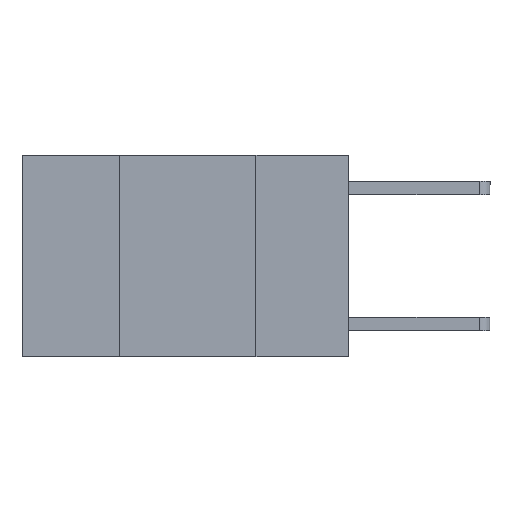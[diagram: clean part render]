
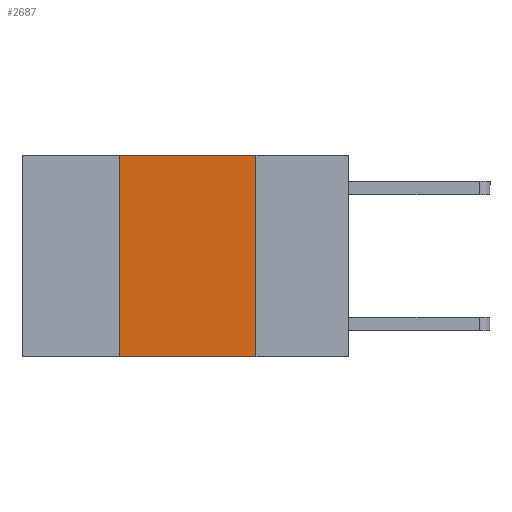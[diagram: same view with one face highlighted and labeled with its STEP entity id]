
A CAD part, left-side view. The second image highlights one B-rep face of the part: STEP entity #2687.
In plain terms, the highlighted planar face has unit normal (-1, 0, 0).
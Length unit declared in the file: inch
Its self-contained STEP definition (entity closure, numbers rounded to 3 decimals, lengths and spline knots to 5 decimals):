
#352 = FACE_OUTER_BOUND ( 'NONE', #5552, .T. ) ;
#398 = ORIENTED_EDGE ( 'NONE', *, *, #6599, .F. ) ;
#625 = VECTOR ( 'NONE', #4652, 39.37008 ) ;
#720 = LINE ( 'NONE', #4434, #6132 ) ;
#852 = LINE ( 'NONE', #4531, #5296 ) ;
#1449 = VERTEX_POINT ( 'NONE', #8248 ) ;
#1647 = CARTESIAN_POINT ( 'NONE',  ( 0., 0.6, 0. ) ) ;
#2238 = VECTOR ( 'NONE', #4436, 39.37008 ) ;
#2485 = LINE ( 'NONE', #7706, #2238 ) ;
#2576 = VERTEX_POINT ( 'NONE', #3418 ) ;
#2687 = ADVANCED_FACE ( 'NONE', ( #352 ), #4977, .F. ) ;
#2700 = CARTESIAN_POINT ( 'NONE',  ( 0., 0.6, -0.37 ) ) ;
#2805 = EDGE_CURVE ( 'NONE', #2576, #2960, #2485, .T. ) ;
#2960 = VERTEX_POINT ( 'NONE', #5774 ) ;
#3195 = CARTESIAN_POINT ( 'NONE',  ( 0., 0.17, -0.37 ) ) ;
#3418 = CARTESIAN_POINT ( 'NONE',  ( 0., 0.42, -0.37 ) ) ;
#3520 = EDGE_CURVE ( 'NONE', #2576, #6836, #7166, .T. ) ;
#3794 = EDGE_CURVE ( 'NONE', #1449, #6836, #720, .T. ) ;
#4040 = AXIS2_PLACEMENT_3D ( 'NONE', #1647, #4310, #6175 ) ;
#4310 = DIRECTION ( 'NONE',  ( 1., 0., 0. ) ) ;
#4434 = CARTESIAN_POINT ( 'NONE',  ( 0., 0.17, 0. ) ) ;
#4436 = DIRECTION ( 'NONE',  ( 0., 0., 1. ) ) ;
#4516 = DIRECTION ( 'NONE',  ( 0., 0., -1. ) ) ;
#4531 = CARTESIAN_POINT ( 'NONE',  ( 0., 0.6, 0. ) ) ;
#4652 = DIRECTION ( 'NONE',  ( 0., -1., 0. ) ) ;
#4977 = PLANE ( 'NONE',  #4040 ) ;
#5296 = VECTOR ( 'NONE', #7090, 39.37008 ) ;
#5552 = EDGE_LOOP ( 'NONE', ( #7351, #398, #6984, #6915 ) ) ;
#5774 = CARTESIAN_POINT ( 'NONE',  ( 0., 0.42, 0. ) ) ;
#6132 = VECTOR ( 'NONE', #4516, 39.37008 ) ;
#6175 = DIRECTION ( 'NONE',  ( 0., 0., -1. ) ) ;
#6599 = EDGE_CURVE ( 'NONE', #2960, #1449, #852, .T. ) ;
#6836 = VERTEX_POINT ( 'NONE', #3195 ) ;
#6915 = ORIENTED_EDGE ( 'NONE', *, *, #3520, .T. ) ;
#6984 = ORIENTED_EDGE ( 'NONE', *, *, #2805, .F. ) ;
#7090 = DIRECTION ( 'NONE',  ( 0., -1., 0. ) ) ;
#7166 = LINE ( 'NONE', #2700, #625 ) ;
#7351 = ORIENTED_EDGE ( 'NONE', *, *, #3794, .F. ) ;
#7706 = CARTESIAN_POINT ( 'NONE',  ( 0., 0.42, 0. ) ) ;
#8248 = CARTESIAN_POINT ( 'NONE',  ( 0., 0.17, 0. ) ) ;
